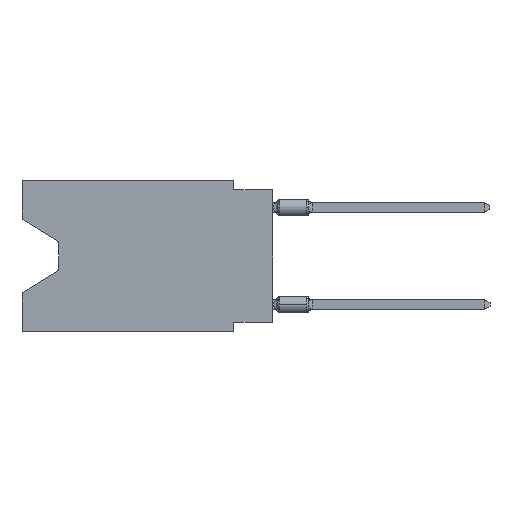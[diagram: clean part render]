
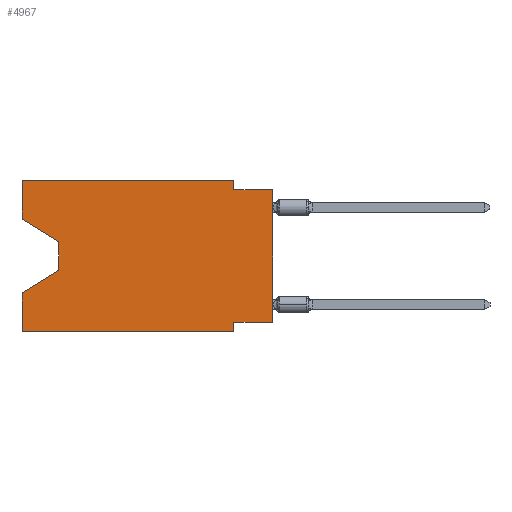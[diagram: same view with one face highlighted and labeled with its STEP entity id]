
A CAD part, left-side view. The second image highlights one B-rep face of the part: STEP entity #4967.
In plain terms, the highlighted planar face has unit normal (-1, 0, 0).
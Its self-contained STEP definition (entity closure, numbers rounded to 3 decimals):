
#501 = DIRECTION ( 'NONE',  ( 0., -0.855, -0.519 ) ) ;
#512 = ORIENTED_EDGE ( 'NONE', *, *, #18194, .T. ) ;
#854 = LINE ( 'NONE', #21750, #2133 ) ;
#1061 = LINE ( 'NONE', #24134, #3899 ) ;
#1350 = VECTOR ( 'NONE', #24591, 1000. ) ;
#1911 = EDGE_CURVE ( 'NONE', #6458, #4149, #1061, .T. ) ;
#1990 = ORIENTED_EDGE ( 'NONE', *, *, #1911, .T. ) ;
#2009 = CARTESIAN_POINT ( 'NONE',  ( 0., 0., -9.271 ) ) ;
#2133 = VECTOR ( 'NONE', #26249, 1000. ) ;
#2701 = DIRECTION ( 'NONE',  ( 0., 0.855, -0.519 ) ) ;
#3353 = EDGE_CURVE ( 'NONE', #25255, #24297, #18466, .T. ) ;
#3551 = VECTOR ( 'NONE', #501, 1000. ) ;
#3658 = CARTESIAN_POINT ( 'NONE',  ( 0., 16.383, 0. ) ) ;
#3899 = VECTOR ( 'NONE', #5430, 1000. ) ;
#4149 = VERTEX_POINT ( 'NONE', #7178 ) ;
#4352 = EDGE_CURVE ( 'NONE', #17482, #16486, #18918, .T. ) ;
#4515 = CARTESIAN_POINT ( 'NONE',  ( 0., 2.54, -0.635 ) ) ;
#4612 = VERTEX_POINT ( 'NONE', #15991 ) ;
#4686 = VECTOR ( 'NONE', #25449, 1000. ) ;
#4967 = ADVANCED_FACE ( 'NONE', ( #24028 ), #5193, .F. ) ;
#5193 = PLANE ( 'NONE',  #25181 ) ;
#5291 = VECTOR ( 'NONE', #22342, 1000. ) ;
#5319 = ORIENTED_EDGE ( 'NONE', *, *, #20447, .T. ) ;
#5430 = DIRECTION ( 'NONE',  ( 0., 0., -1. ) ) ;
#5452 = EDGE_CURVE ( 'NONE', #4612, #11284, #17853, .T. ) ;
#5689 = DIRECTION ( 'NONE',  ( 0., 0., 1. ) ) ;
#5749 = EDGE_CURVE ( 'NONE', #25675, #11284, #854, .T. ) ;
#5824 = ORIENTED_EDGE ( 'NONE', *, *, #14142, .F. ) ;
#6342 = LINE ( 'NONE', #10585, #4686 ) ;
#6458 = VERTEX_POINT ( 'NONE', #25105 ) ;
#6721 = DIRECTION ( 'NONE',  ( 0., 1., 0. ) ) ;
#7178 = CARTESIAN_POINT ( 'NONE',  ( 0., 13.97, -5.893 ) ) ;
#8085 = VECTOR ( 'NONE', #2701, 1000. ) ;
#8654 = DIRECTION ( 'NONE',  ( 0., 0., -1. ) ) ;
#9139 = ORIENTED_EDGE ( 'NONE', *, *, #25260, .F. ) ;
#9140 = CARTESIAN_POINT ( 'NONE',  ( 0., 16.383, -9.906 ) ) ;
#9439 = CARTESIAN_POINT ( 'NONE',  ( 0., 16.383, -7.36 ) ) ;
#9798 = LINE ( 'NONE', #21943, #11722 ) ;
#10585 = CARTESIAN_POINT ( 'NONE',  ( 0., 0., -0.635 ) ) ;
#10714 = VERTEX_POINT ( 'NONE', #17507 ) ;
#10974 = ORIENTED_EDGE ( 'NONE', *, *, #16846, .T. ) ;
#11158 = LINE ( 'NONE', #17299, #8085 ) ;
#11206 = CARTESIAN_POINT ( 'NONE',  ( 0., 16.383, 0. ) ) ;
#11284 = VERTEX_POINT ( 'NONE', #18523 ) ;
#11343 = DIRECTION ( 'NONE',  ( 1., 0., 0. ) ) ;
#11722 = VECTOR ( 'NONE', #5689, 1000. ) ;
#13230 = EDGE_CURVE ( 'NONE', #24297, #17482, #17651, .T. ) ;
#13276 = LINE ( 'NONE', #23372, #19532 ) ;
#14104 = CARTESIAN_POINT ( 'NONE',  ( 0., 16.383, 0. ) ) ;
#14142 = EDGE_CURVE ( 'NONE', #25675, #18660, #9798, .T. ) ;
#14221 = CARTESIAN_POINT ( 'NONE',  ( 0., 2.54, 0. ) ) ;
#14794 = CARTESIAN_POINT ( 'NONE',  ( 0., 2.54, 0. ) ) ;
#15193 = DIRECTION ( 'NONE',  ( 0., -1., 0. ) ) ;
#15356 = EDGE_LOOP ( 'NONE', ( #10974, #1990, #5319, #5824, #21539, #26477, #9139, #512, #23192, #15858, #16887, #22856 ) ) ;
#15858 = ORIENTED_EDGE ( 'NONE', *, *, #4352, .F. ) ;
#15991 = CARTESIAN_POINT ( 'NONE',  ( 0., 2.54, -9.271 ) ) ;
#16486 = VERTEX_POINT ( 'NONE', #4515 ) ;
#16735 = CARTESIAN_POINT ( 'NONE',  ( 0., 16.383, 0. ) ) ;
#16846 = EDGE_CURVE ( 'NONE', #25255, #6458, #23582, .T. ) ;
#16887 = ORIENTED_EDGE ( 'NONE', *, *, #13230, .F. ) ;
#17299 = CARTESIAN_POINT ( 'NONE',  ( 0., 13.97, -5.893 ) ) ;
#17482 = VERTEX_POINT ( 'NONE', #14221 ) ;
#17507 = CARTESIAN_POINT ( 'NONE',  ( 0., 0., -0.635 ) ) ;
#17651 = LINE ( 'NONE', #16735, #18593 ) ;
#17853 = LINE ( 'NONE', #22860, #23021 ) ;
#18194 = EDGE_CURVE ( 'NONE', #23135, #10714, #24375, .T. ) ;
#18253 = CARTESIAN_POINT ( 'NONE',  ( 0., 0., 0. ) ) ;
#18466 = LINE ( 'NONE', #14104, #1350 ) ;
#18523 = CARTESIAN_POINT ( 'NONE',  ( 0., 2.54, -9.906 ) ) ;
#18593 = VECTOR ( 'NONE', #15193, 1000. ) ;
#18623 = CARTESIAN_POINT ( 'NONE',  ( 0., 16.383, -2.546 ) ) ;
#18660 = VERTEX_POINT ( 'NONE', #9439 ) ;
#18918 = LINE ( 'NONE', #14794, #23630 ) ;
#19532 = VECTOR ( 'NONE', #6721, 1000. ) ;
#20447 = EDGE_CURVE ( 'NONE', #4149, #18660, #11158, .T. ) ;
#21539 = ORIENTED_EDGE ( 'NONE', *, *, #5749, .T. ) ;
#21750 = CARTESIAN_POINT ( 'NONE',  ( 0., 16.383, -9.906 ) ) ;
#21943 = CARTESIAN_POINT ( 'NONE',  ( 0., 16.383, 0. ) ) ;
#22342 = DIRECTION ( 'NONE',  ( 0., 0., 1. ) ) ;
#22856 = ORIENTED_EDGE ( 'NONE', *, *, #3353, .F. ) ;
#22860 = CARTESIAN_POINT ( 'NONE',  ( 0., 2.54, -9.906 ) ) ;
#23021 = VECTOR ( 'NONE', #24385, 1000. ) ;
#23135 = VERTEX_POINT ( 'NONE', #2009 ) ;
#23192 = ORIENTED_EDGE ( 'NONE', *, *, #24722, .F. ) ;
#23372 = CARTESIAN_POINT ( 'NONE',  ( 0., 0., -9.271 ) ) ;
#23582 = LINE ( 'NONE', #25358, #3551 ) ;
#23630 = VECTOR ( 'NONE', #8654, 1000. ) ;
#24028 = FACE_OUTER_BOUND ( 'NONE', #15356, .T. ) ;
#24134 = CARTESIAN_POINT ( 'NONE',  ( 0., 13.97, -4.013 ) ) ;
#24297 = VERTEX_POINT ( 'NONE', #3658 ) ;
#24375 = LINE ( 'NONE', #18253, #5291 ) ;
#24385 = DIRECTION ( 'NONE',  ( 0., 0., -1. ) ) ;
#24591 = DIRECTION ( 'NONE',  ( 0., 0., 1. ) ) ;
#24722 = EDGE_CURVE ( 'NONE', #16486, #10714, #6342, .T. ) ;
#25105 = CARTESIAN_POINT ( 'NONE',  ( 0., 13.97, -4.013 ) ) ;
#25181 = AXIS2_PLACEMENT_3D ( 'NONE', #11206, #11343, #26206 ) ;
#25255 = VERTEX_POINT ( 'NONE', #18623 ) ;
#25260 = EDGE_CURVE ( 'NONE', #23135, #4612, #13276, .T. ) ;
#25358 = CARTESIAN_POINT ( 'NONE',  ( 0., 16.383, -2.546 ) ) ;
#25449 = DIRECTION ( 'NONE',  ( 0., -1., 0. ) ) ;
#25675 = VERTEX_POINT ( 'NONE', #9140 ) ;
#26206 = DIRECTION ( 'NONE',  ( 0., 0., -1. ) ) ;
#26249 = DIRECTION ( 'NONE',  ( 0., -1., 0. ) ) ;
#26477 = ORIENTED_EDGE ( 'NONE', *, *, #5452, .F. ) ;
